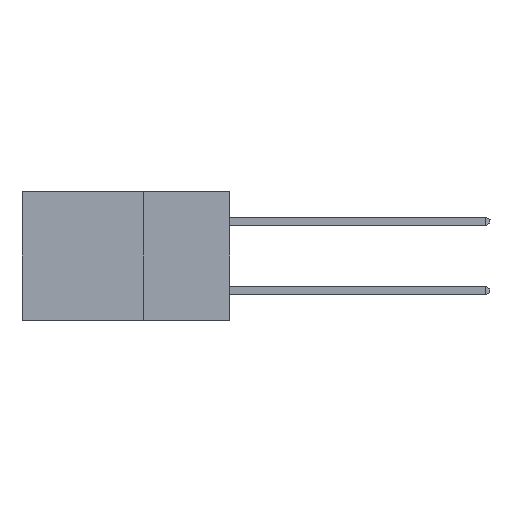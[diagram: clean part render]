
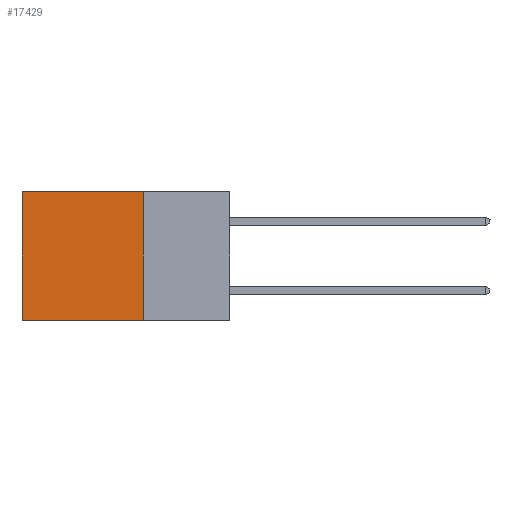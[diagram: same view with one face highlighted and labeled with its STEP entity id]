
A CAD part, left-side view. The second image highlights one B-rep face of the part: STEP entity #17429.
In plain terms, the highlighted planar face has unit normal (-1, 0, 0).
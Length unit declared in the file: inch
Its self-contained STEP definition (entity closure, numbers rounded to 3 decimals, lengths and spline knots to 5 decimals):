
#196 = CARTESIAN_POINT ( 'NONE',  ( 0.298, 0.25, -0.37 ) ) ;
#424 = LINE ( 'NONE', #8283, #5226 ) ;
#1133 = LINE ( 'NONE', #196, #20772 ) ;
#2794 = DIRECTION ( 'NONE',  ( 0., 0., -1. ) ) ;
#3893 = EDGE_CURVE ( 'NONE', #10438, #22561, #1133, .T. ) ;
#4333 = EDGE_LOOP ( 'NONE', ( #19568, #22366, #13812, #18763 ) ) ;
#4990 = VECTOR ( 'NONE', #2794, 39.37008 ) ;
#5226 = VECTOR ( 'NONE', #7762, 39.37008 ) ;
#7492 = EDGE_CURVE ( 'NONE', #22721, #10438, #8564, .T. ) ;
#7762 = DIRECTION ( 'NONE',  ( 0., 1., 0. ) ) ;
#8090 = EDGE_CURVE ( 'NONE', #22721, #13775, #424, .T. ) ;
#8283 = CARTESIAN_POINT ( 'NONE',  ( 0.298, 0.25, 0. ) ) ;
#8421 = CARTESIAN_POINT ( 'NONE',  ( 0.298, 0.25, 0. ) ) ;
#8564 = LINE ( 'NONE', #12967, #13278 ) ;
#9714 = CARTESIAN_POINT ( 'NONE',  ( 0.298, 0.25, -0.37 ) ) ;
#10281 = DIRECTION ( 'NONE',  ( 0., 0., -1. ) ) ;
#10353 = LINE ( 'NONE', #24890, #4990 ) ;
#10417 = DIRECTION ( 'NONE',  ( 1., 0., 0. ) ) ;
#10438 = VERTEX_POINT ( 'NONE', #9714 ) ;
#12967 = CARTESIAN_POINT ( 'NONE',  ( 0.298, 0.25, 0. ) ) ;
#13278 = VECTOR ( 'NONE', #10281, 39.37008 ) ;
#13775 = VERTEX_POINT ( 'NONE', #18084 ) ;
#13812 = ORIENTED_EDGE ( 'NONE', *, *, #7492, .F. ) ;
#14171 = DIRECTION ( 'NONE',  ( 0., 1., 0. ) ) ;
#14772 = CARTESIAN_POINT ( 'NONE',  ( 0.298, 0.25, 0. ) ) ;
#17429 = ADVANCED_FACE ( 'NONE', ( #20268 ), #20524, .F. ) ;
#18084 = CARTESIAN_POINT ( 'NONE',  ( 0.298, 0.6, 0. ) ) ;
#18763 = ORIENTED_EDGE ( 'NONE', *, *, #8090, .T. ) ;
#18920 = EDGE_CURVE ( 'NONE', #13775, #22561, #10353, .T. ) ;
#19568 = ORIENTED_EDGE ( 'NONE', *, *, #18920, .T. ) ;
#20268 = FACE_OUTER_BOUND ( 'NONE', #4333, .T. ) ;
#20524 = PLANE ( 'NONE',  #21941 ) ;
#20772 = VECTOR ( 'NONE', #14171, 39.37008 ) ;
#21941 = AXIS2_PLACEMENT_3D ( 'NONE', #8421, #10417, #24504 ) ;
#22366 = ORIENTED_EDGE ( 'NONE', *, *, #3893, .F. ) ;
#22561 = VERTEX_POINT ( 'NONE', #25236 ) ;
#22721 = VERTEX_POINT ( 'NONE', #14772 ) ;
#24504 = DIRECTION ( 'NONE',  ( 0., 0., -1. ) ) ;
#24890 = CARTESIAN_POINT ( 'NONE',  ( 0.298, 0.6, 0. ) ) ;
#25236 = CARTESIAN_POINT ( 'NONE',  ( 0.298, 0.6, -0.37 ) ) ;
